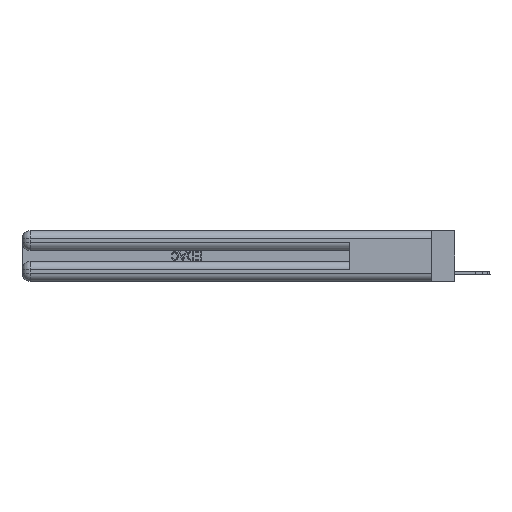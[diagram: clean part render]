
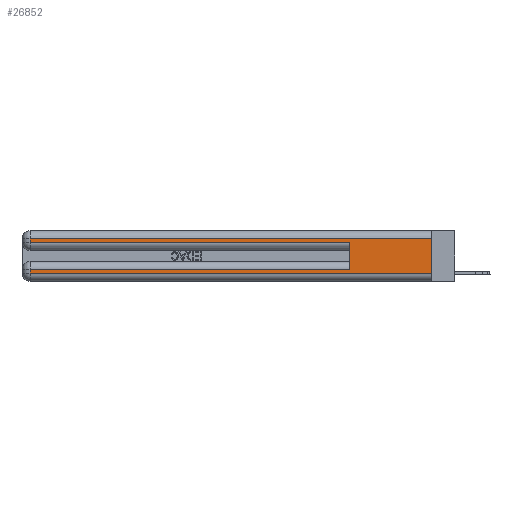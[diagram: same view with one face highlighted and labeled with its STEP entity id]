
A CAD part, left-side view. The second image highlights one B-rep face of the part: STEP entity #26852.
In plain terms, the highlighted planar face has unit normal (-1, 0, 0).
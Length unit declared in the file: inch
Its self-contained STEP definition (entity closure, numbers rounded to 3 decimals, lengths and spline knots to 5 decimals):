
#118 = CARTESIAN_POINT ( 'NONE',  ( 0., 0., 0.06 ) ) ;
#342 = VERTEX_POINT ( 'NONE', #6325 ) ;
#548 = CARTESIAN_POINT ( 'NONE',  ( 0., 0., 0.31 ) ) ;
#895 = VERTEX_POINT ( 'NONE', #11280 ) ;
#1911 = LINE ( 'NONE', #20939, #20288 ) ;
#2620 = CARTESIAN_POINT ( 'NONE',  ( 0., 0., 0.06 ) ) ;
#2686 = EDGE_CURVE ( 'NONE', #7109, #3872, #17098, .T. ) ;
#2762 = LINE ( 'NONE', #2620, #18919 ) ;
#3212 = CARTESIAN_POINT ( 'NONE',  ( 0., 0., 0.37 ) ) ;
#3232 = ORIENTED_EDGE ( 'NONE', *, *, #19074, .F. ) ;
#3297 = VECTOR ( 'NONE', #24644, 39.37008 ) ;
#3872 = VERTEX_POINT ( 'NONE', #12994 ) ;
#4535 = EDGE_CURVE ( 'NONE', #7951, #895, #18579, .T. ) ;
#5319 = PLANE ( 'NONE',  #8989 ) ;
#5697 = VECTOR ( 'NONE', #22172, 39.37008 ) ;
#5982 = EDGE_LOOP ( 'NONE', ( #16870, #20966, #6101, #18736, #3232, #21890, #8205, #13897 ) ) ;
#6101 = ORIENTED_EDGE ( 'NONE', *, *, #21850, .T. ) ;
#6255 = VECTOR ( 'NONE', #27244, 39.37008 ) ;
#6325 = CARTESIAN_POINT ( 'NONE',  ( 0., 2.94, 0.285 ) ) ;
#7109 = VERTEX_POINT ( 'NONE', #548 ) ;
#7185 = CARTESIAN_POINT ( 'NONE',  ( 0., 0., 0.37 ) ) ;
#7235 = CARTESIAN_POINT ( 'NONE',  ( 0., 2.94, 0.085 ) ) ;
#7288 = DIRECTION ( 'NONE',  ( 0., -1., 0. ) ) ;
#7454 = EDGE_CURVE ( 'NONE', #11451, #7951, #17966, .T. ) ;
#7951 = VERTEX_POINT ( 'NONE', #7235 ) ;
#8061 = LINE ( 'NONE', #25271, #6255 ) ;
#8205 = ORIENTED_EDGE ( 'NONE', *, *, #4535, .T. ) ;
#8989 = AXIS2_PLACEMENT_3D ( 'NONE', #7185, #24375, #11781 ) ;
#11112 = CARTESIAN_POINT ( 'NONE',  ( 0., 0., 0.31 ) ) ;
#11280 = CARTESIAN_POINT ( 'NONE',  ( 0., 2.94, 0.06 ) ) ;
#11451 = VERTEX_POINT ( 'NONE', #20730 ) ;
#11575 = EDGE_CURVE ( 'NONE', #7109, #21431, #13507, .T. ) ;
#11781 = DIRECTION ( 'NONE',  ( 0., 0., -1. ) ) ;
#11789 = CARTESIAN_POINT ( 'NONE',  ( 0., 2.94, 0.37 ) ) ;
#11935 = DIRECTION ( 'NONE',  ( 0., 0., -1. ) ) ;
#12994 = CARTESIAN_POINT ( 'NONE',  ( 0., 2.94, 0.31 ) ) ;
#13507 = LINE ( 'NONE', #3212, #3297 ) ;
#13775 = FACE_OUTER_BOUND ( 'NONE', #5982, .T. ) ;
#13846 = LINE ( 'NONE', #26985, #15175 ) ;
#13873 = VECTOR ( 'NONE', #19945, 39.37008 ) ;
#13897 = ORIENTED_EDGE ( 'NONE', *, *, #21572, .T. ) ;
#14842 = DIRECTION ( 'NONE',  ( 0., 0., -1. ) ) ;
#15175 = VECTOR ( 'NONE', #20483, 39.37008 ) ;
#16695 = EDGE_CURVE ( 'NONE', #342, #17836, #13846, .T. ) ;
#16798 = CARTESIAN_POINT ( 'NONE',  ( 0., 0.6, 0.285 ) ) ;
#16870 = ORIENTED_EDGE ( 'NONE', *, *, #11575, .F. ) ;
#17098 = LINE ( 'NONE', #11112, #5697 ) ;
#17836 = VERTEX_POINT ( 'NONE', #16798 ) ;
#17966 = LINE ( 'NONE', #26165, #13873 ) ;
#18579 = LINE ( 'NONE', #11789, #24223 ) ;
#18736 = ORIENTED_EDGE ( 'NONE', *, *, #16695, .T. ) ;
#18919 = VECTOR ( 'NONE', #7288, 39.37008 ) ;
#19074 = EDGE_CURVE ( 'NONE', #11451, #17836, #8061, .T. ) ;
#19945 = DIRECTION ( 'NONE',  ( 0., 1., 0. ) ) ;
#20288 = VECTOR ( 'NONE', #14842, 39.37008 ) ;
#20483 = DIRECTION ( 'NONE',  ( 0., -1., 0. ) ) ;
#20730 = CARTESIAN_POINT ( 'NONE',  ( 0., 0.6, 0.085 ) ) ;
#20939 = CARTESIAN_POINT ( 'NONE',  ( 0., 2.94, 0.37 ) ) ;
#20966 = ORIENTED_EDGE ( 'NONE', *, *, #2686, .T. ) ;
#21431 = VERTEX_POINT ( 'NONE', #118 ) ;
#21572 = EDGE_CURVE ( 'NONE', #895, #21431, #2762, .T. ) ;
#21850 = EDGE_CURVE ( 'NONE', #3872, #342, #1911, .T. ) ;
#21890 = ORIENTED_EDGE ( 'NONE', *, *, #7454, .T. ) ;
#22172 = DIRECTION ( 'NONE',  ( 0., 1., 0. ) ) ;
#24223 = VECTOR ( 'NONE', #11935, 39.37008 ) ;
#24375 = DIRECTION ( 'NONE',  ( 1., 0., 0. ) ) ;
#24644 = DIRECTION ( 'NONE',  ( 0., 0., -1. ) ) ;
#25271 = CARTESIAN_POINT ( 'NONE',  ( 0., 0.6, 0.145 ) ) ;
#26165 = CARTESIAN_POINT ( 'NONE',  ( 0., 0., 0.085 ) ) ;
#26852 = ADVANCED_FACE ( 'NONE', ( #13775 ), #5319, .F. ) ;
#26985 = CARTESIAN_POINT ( 'NONE',  ( 0., 0., 0.285 ) ) ;
#27244 = DIRECTION ( 'NONE',  ( 0., 0., 1. ) ) ;
